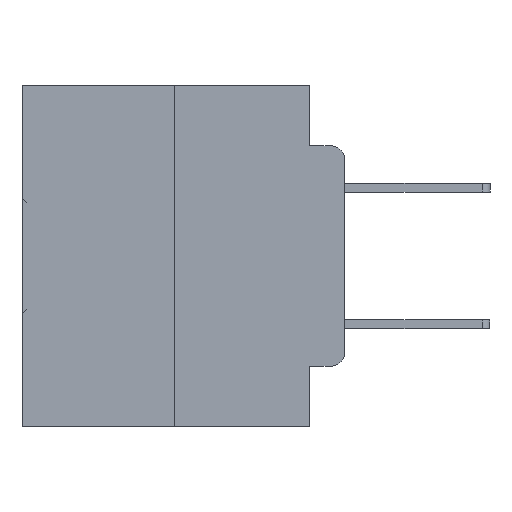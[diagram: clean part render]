
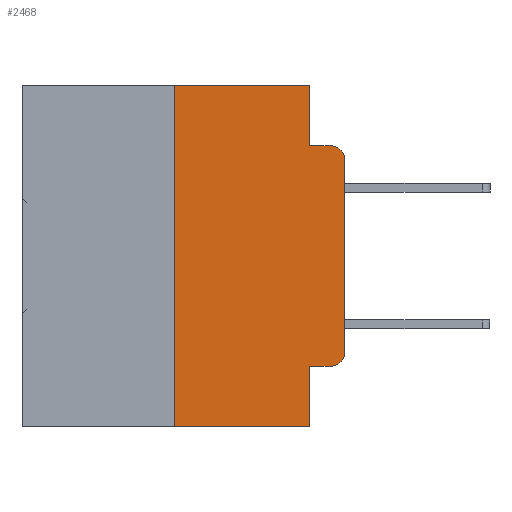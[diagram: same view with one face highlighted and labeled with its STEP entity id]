
A CAD part, left-side view. The second image highlights one B-rep face of the part: STEP entity #2468.
In plain terms, the highlighted planar face has unit normal (-1, 0, 0).
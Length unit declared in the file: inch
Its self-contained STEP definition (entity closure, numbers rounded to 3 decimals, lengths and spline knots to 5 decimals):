
#813 = CIRCLE ( 'NONE', #5037, 0.02 ) ;
#1089 = EDGE_CURVE ( 'NONE', #30699, #31347, #813, .T. ) ;
#1582 = CARTESIAN_POINT ( 'NONE',  ( 0., 0.02, -0.1085 ) ) ;
#1588 = LINE ( 'NONE', #3566, #7558 ) ;
#2162 = DIRECTION ( 'NONE',  ( 0., -1., 0. ) ) ;
#2468 = ADVANCED_FACE ( 'NONE', ( #31679 ), #27599, .F. ) ;
#3566 = CARTESIAN_POINT ( 'NONE',  ( 0., 0., 0. ) ) ;
#3650 = CARTESIAN_POINT ( 'NONE',  ( 0., 0., -0.3915 ) ) ;
#3838 = VERTEX_POINT ( 'NONE', #10997 ) ;
#4022 = CARTESIAN_POINT ( 'NONE',  ( 0., 0.051, 0. ) ) ;
#4167 = DIRECTION ( 'NONE',  ( 0., 0., -1. ) ) ;
#4291 = CARTESIAN_POINT ( 'NONE',  ( 0., 0.051, 0. ) ) ;
#4885 = CARTESIAN_POINT ( 'NONE',  ( 0., 0.02, -0.4115 ) ) ;
#5037 = AXIS2_PLACEMENT_3D ( 'NONE', #1582, #19241, #4167 ) ;
#5248 = ORIENTED_EDGE ( 'NONE', *, *, #21137, .T. ) ;
#5408 = VECTOR ( 'NONE', #19843, 39.37008 ) ;
#5522 = EDGE_CURVE ( 'NONE', #24037, #21486, #12176, .T. ) ;
#5788 = DIRECTION ( 'NONE',  ( 0., -1., 0. ) ) ;
#5812 = CARTESIAN_POINT ( 'NONE',  ( 0., 0.02, -0.0885 ) ) ;
#6049 = EDGE_CURVE ( 'NONE', #30384, #21333, #22316, .T. ) ;
#6879 = EDGE_CURVE ( 'NONE', #24037, #11050, #11290, .T. ) ;
#7558 = VECTOR ( 'NONE', #8620, 39.37008 ) ;
#7759 = CIRCLE ( 'NONE', #31599, 0.02 ) ;
#7843 = CARTESIAN_POINT ( 'NONE',  ( 0., 0.473, 0. ) ) ;
#8276 = CARTESIAN_POINT ( 'NONE',  ( 0., 0.051, -0.0885 ) ) ;
#8620 = DIRECTION ( 'NONE',  ( 0., 0., 1. ) ) ;
#8938 = EDGE_CURVE ( 'NONE', #11050, #21951, #7759, .T. ) ;
#9089 = ORIENTED_EDGE ( 'NONE', *, *, #25228, .F. ) ;
#9458 = DIRECTION ( 'NONE',  ( -1., 0., 0. ) ) ;
#10341 = ORIENTED_EDGE ( 'NONE', *, *, #6879, .T. ) ;
#10544 = CARTESIAN_POINT ( 'NONE',  ( 0., 0.051, -0.0885 ) ) ;
#10997 = CARTESIAN_POINT ( 'NONE',  ( 0., 0.25, 0. ) ) ;
#11032 = ORIENTED_EDGE ( 'NONE', *, *, #29593, .T. ) ;
#11050 = VERTEX_POINT ( 'NONE', #4885 ) ;
#11290 = LINE ( 'NONE', #17306, #5408 ) ;
#11699 = CARTESIAN_POINT ( 'NONE',  ( 0., 0.051, 0. ) ) ;
#12176 = LINE ( 'NONE', #4291, #31098 ) ;
#12222 = CARTESIAN_POINT ( 'NONE',  ( 0., 0.473, -0.5 ) ) ;
#14160 = DIRECTION ( 'NONE',  ( 0., 0., -1. ) ) ;
#15648 = VECTOR ( 'NONE', #14160, 39.37008 ) ;
#15696 = CARTESIAN_POINT ( 'NONE',  ( 0., 0., -0.1085 ) ) ;
#15987 = AXIS2_PLACEMENT_3D ( 'NONE', #22399, #28917, #17017 ) ;
#17017 = DIRECTION ( 'NONE',  ( 0., 0., -1. ) ) ;
#17248 = VECTOR ( 'NONE', #5788, 39.37008 ) ;
#17306 = CARTESIAN_POINT ( 'NONE',  ( 0., 0.051, -0.4115 ) ) ;
#17529 = ORIENTED_EDGE ( 'NONE', *, *, #24799, .F. ) ;
#18515 = VECTOR ( 'NONE', #28393, 39.37008 ) ;
#19241 = DIRECTION ( 'NONE',  ( -1., 0., 0. ) ) ;
#19245 = ORIENTED_EDGE ( 'NONE', *, *, #1089, .T. ) ;
#19843 = DIRECTION ( 'NONE',  ( 0., -1., 0. ) ) ;
#20929 = VECTOR ( 'NONE', #2162, 39.37008 ) ;
#20995 = CARTESIAN_POINT ( 'NONE',  ( 0., 0.25, 0. ) ) ;
#21137 = EDGE_CURVE ( 'NONE', #22486, #21486, #28226, .T. ) ;
#21333 = VERTEX_POINT ( 'NONE', #10544 ) ;
#21486 = VERTEX_POINT ( 'NONE', #23672 ) ;
#21951 = VERTEX_POINT ( 'NONE', #3650 ) ;
#22313 = CARTESIAN_POINT ( 'NONE',  ( 0., 0.051, -0.4115 ) ) ;
#22316 = LINE ( 'NONE', #4022, #15648 ) ;
#22399 = CARTESIAN_POINT ( 'NONE',  ( 0., 0.473, 0. ) ) ;
#22486 = VERTEX_POINT ( 'NONE', #25827 ) ;
#22505 = EDGE_CURVE ( 'NONE', #22486, #3838, #32289, .T. ) ;
#23672 = CARTESIAN_POINT ( 'NONE',  ( 0., 0.051, -0.5 ) ) ;
#23862 = LINE ( 'NONE', #8276, #17248 ) ;
#24037 = VERTEX_POINT ( 'NONE', #22313 ) ;
#24466 = CARTESIAN_POINT ( 'NONE',  ( 0., 0.02, -0.3915 ) ) ;
#24799 = EDGE_CURVE ( 'NONE', #21333, #31347, #23862, .T. ) ;
#25228 = EDGE_CURVE ( 'NONE', #3838, #30384, #26894, .T. ) ;
#25827 = CARTESIAN_POINT ( 'NONE',  ( 0., 0.25, -0.5 ) ) ;
#25959 = ORIENTED_EDGE ( 'NONE', *, *, #22505, .F. ) ;
#26791 = DIRECTION ( 'NONE',  ( 0., 0., -1. ) ) ;
#26894 = LINE ( 'NONE', #7843, #30276 ) ;
#26913 = DIRECTION ( 'NONE',  ( 0., 0., -1. ) ) ;
#27502 = ORIENTED_EDGE ( 'NONE', *, *, #6049, .F. ) ;
#27599 = PLANE ( 'NONE',  #15987 ) ;
#28226 = LINE ( 'NONE', #12222, #20929 ) ;
#28393 = DIRECTION ( 'NONE',  ( 0., 0., 1. ) ) ;
#28917 = DIRECTION ( 'NONE',  ( 1., 0., 0. ) ) ;
#29385 = ORIENTED_EDGE ( 'NONE', *, *, #8938, .T. ) ;
#29456 = EDGE_LOOP ( 'NONE', ( #11032, #19245, #17529, #27502, #9089, #25959, #5248, #30860, #10341, #29385 ) ) ;
#29593 = EDGE_CURVE ( 'NONE', #21951, #30699, #1588, .T. ) ;
#30079 = DIRECTION ( 'NONE',  ( 0., -1., 0. ) ) ;
#30276 = VECTOR ( 'NONE', #30079, 39.37008 ) ;
#30384 = VERTEX_POINT ( 'NONE', #11699 ) ;
#30699 = VERTEX_POINT ( 'NONE', #15696 ) ;
#30860 = ORIENTED_EDGE ( 'NONE', *, *, #5522, .F. ) ;
#31098 = VECTOR ( 'NONE', #26791, 39.37008 ) ;
#31347 = VERTEX_POINT ( 'NONE', #5812 ) ;
#31599 = AXIS2_PLACEMENT_3D ( 'NONE', #24466, #9458, #26913 ) ;
#31679 = FACE_OUTER_BOUND ( 'NONE', #29456, .T. ) ;
#32289 = LINE ( 'NONE', #20995, #18515 ) ;
